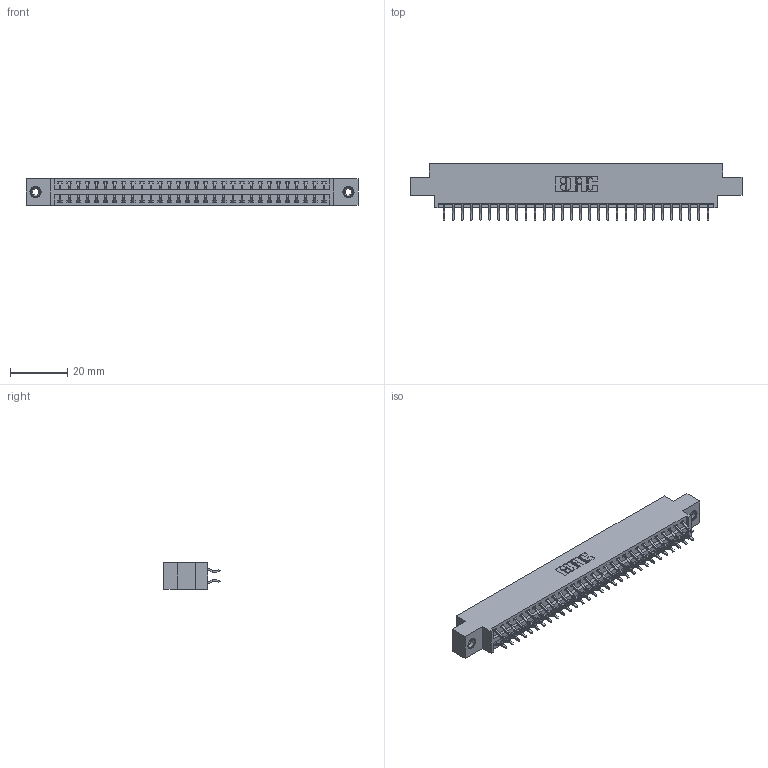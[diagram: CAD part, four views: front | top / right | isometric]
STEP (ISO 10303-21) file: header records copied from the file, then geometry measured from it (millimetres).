
FILE_DESCRIPTION (( 'STEP AP203' ), '1' );
FILE_NAME ('346-060-556-808.STEP', '2022-05-21T12:10:19', ( '' ), ( '' ), 'SwSTEP 2.0', 'SolidWorks 2020', '' );
FILE_SCHEMA (( 'CONFIG_CONTROL_DESIGN' ));
Length unit declared in the file: inch
Products named in the file (4): 345-250-001_345-250-003-102; 345-292-001_556 Tail; 346 Part_0.170 Offset - 0.156 Dia-TI; 346-060-556-808
Assembly tree (63 placements, depth 2):
  346-060-556-808
    346 Part_0.170 Offset - 0.156 Dia-TI
    345-292-001_556 Tail  x60
    345-250-001_345-250-003-102  x2
Bounding box: 115.82 x 19.57 x 9.4 mm (x, y, z)
Volume: 11037.6 mm3; surface area: 15127.2 mm2
Topology: 63 solids, 63 shells, 3666 faces, 10857 edges, 7150 vertices
Faces by surface type: plane 2452, cylinder 1198, cone 12, torus 4
Entity records: 22732 total; most frequent: CARTESIAN_POINT 3763, ORIENTED_EDGE 3678, DIRECTION 3381, EDGE_CURVE 1839, LINE 1559, VECTOR 1559, VERTEX_POINT 1220, AXIS2_PLACEMENT_3D 911
